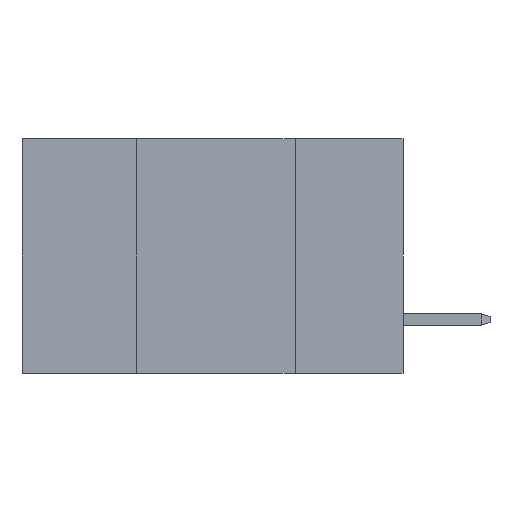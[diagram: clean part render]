
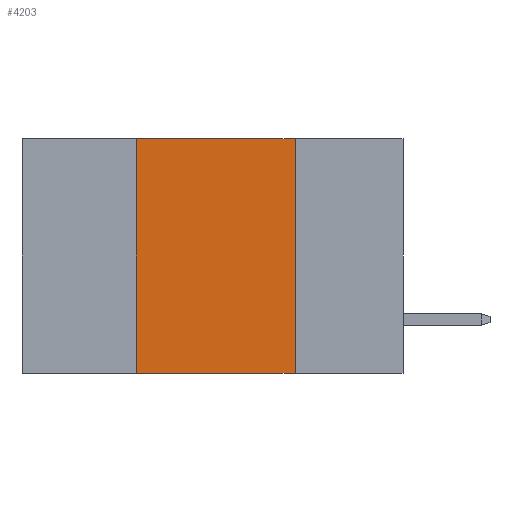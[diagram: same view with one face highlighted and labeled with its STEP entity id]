
A CAD part, left-side view. The second image highlights one B-rep face of the part: STEP entity #4203.
In plain terms, the highlighted planar face has unit normal (-1, 0, 0).
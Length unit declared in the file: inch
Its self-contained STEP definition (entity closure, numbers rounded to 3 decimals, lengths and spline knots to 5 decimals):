
#455 = CARTESIAN_POINT ( 'NONE',  ( 0., 0.17, -0.37 ) ) ;
#500 = LINE ( 'NONE', #9693, #4790 ) ;
#523 = EDGE_LOOP ( 'NONE', ( #4575, #9445, #2507, #7825 ) ) ;
#953 = VECTOR ( 'NONE', #10784, 39.37008 ) ;
#1496 = VERTEX_POINT ( 'NONE', #4464 ) ;
#1686 = DIRECTION ( 'NONE',  ( 0., 0., -1. ) ) ;
#1928 = DIRECTION ( 'NONE',  ( 0., 0., 1. ) ) ;
#2417 = CARTESIAN_POINT ( 'NONE',  ( 0., 0.42, -0.37 ) ) ;
#2507 = ORIENTED_EDGE ( 'NONE', *, *, #7830, .F. ) ;
#2799 = LINE ( 'NONE', #4394, #8633 ) ;
#3821 = DIRECTION ( 'NONE',  ( 0., -1., 0. ) ) ;
#4086 = CARTESIAN_POINT ( 'NONE',  ( 0., 0.17, 0. ) ) ;
#4129 = CARTESIAN_POINT ( 'NONE',  ( 0., 0.6, 0. ) ) ;
#4203 = ADVANCED_FACE ( 'NONE', ( #10124 ), #4965, .F. ) ;
#4346 = CARTESIAN_POINT ( 'NONE',  ( 0., 0.17, 0. ) ) ;
#4394 = CARTESIAN_POINT ( 'NONE',  ( 0., 0.42, 0. ) ) ;
#4464 = CARTESIAN_POINT ( 'NONE',  ( 0., 0.42, 0. ) ) ;
#4575 = ORIENTED_EDGE ( 'NONE', *, *, #4838, .F. ) ;
#4790 = VECTOR ( 'NONE', #3821, 39.37008 ) ;
#4838 = EDGE_CURVE ( 'NONE', #8211, #9318, #6003, .T. ) ;
#4965 = PLANE ( 'NONE',  #8419 ) ;
#5070 = VERTEX_POINT ( 'NONE', #2417 ) ;
#5808 = VECTOR ( 'NONE', #10217, 39.37008 ) ;
#6003 = LINE ( 'NONE', #4346, #5808 ) ;
#6614 = DIRECTION ( 'NONE',  ( 1., 0., 0. ) ) ;
#7326 = EDGE_CURVE ( 'NONE', #5070, #9318, #9912, .T. ) ;
#7440 = CARTESIAN_POINT ( 'NONE',  ( 0., 0.6, -0.37 ) ) ;
#7825 = ORIENTED_EDGE ( 'NONE', *, *, #7326, .T. ) ;
#7830 = EDGE_CURVE ( 'NONE', #5070, #1496, #2799, .T. ) ;
#8211 = VERTEX_POINT ( 'NONE', #4086 ) ;
#8419 = AXIS2_PLACEMENT_3D ( 'NONE', #4129, #6614, #1686 ) ;
#8633 = VECTOR ( 'NONE', #1928, 39.37008 ) ;
#9318 = VERTEX_POINT ( 'NONE', #455 ) ;
#9349 = EDGE_CURVE ( 'NONE', #1496, #8211, #500, .T. ) ;
#9445 = ORIENTED_EDGE ( 'NONE', *, *, #9349, .F. ) ;
#9693 = CARTESIAN_POINT ( 'NONE',  ( 0., 0.6, 0. ) ) ;
#9912 = LINE ( 'NONE', #7440, #953 ) ;
#10124 = FACE_OUTER_BOUND ( 'NONE', #523, .T. ) ;
#10217 = DIRECTION ( 'NONE',  ( 0., 0., -1. ) ) ;
#10784 = DIRECTION ( 'NONE',  ( 0., -1., 0. ) ) ;
